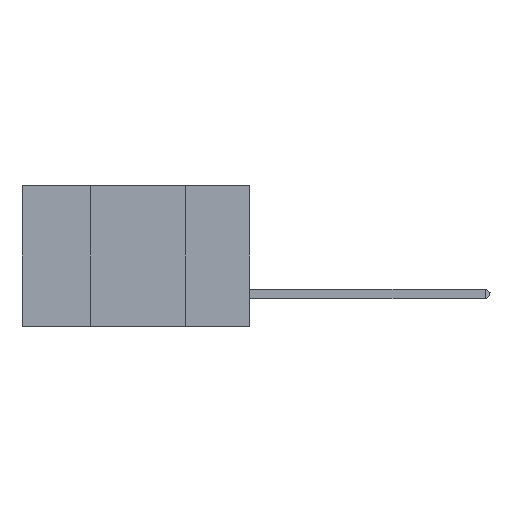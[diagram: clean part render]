
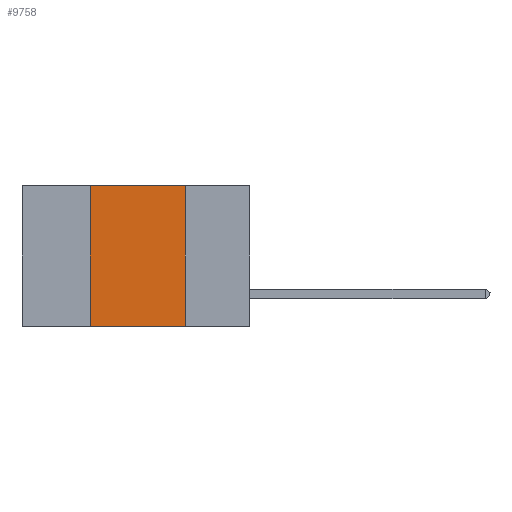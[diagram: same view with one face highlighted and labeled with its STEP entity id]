
A CAD part, left-side view. The second image highlights one B-rep face of the part: STEP entity #9758.
In plain terms, the highlighted planar face has unit normal (-1, 0, 0).
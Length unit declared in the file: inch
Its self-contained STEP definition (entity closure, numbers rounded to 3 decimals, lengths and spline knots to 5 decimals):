
#1117 = DIRECTION ( 'NONE',  ( 0., -1., 0. ) ) ;
#2563 = DIRECTION ( 'NONE',  ( 1., 0., 0. ) ) ;
#5651 = EDGE_CURVE ( 'NONE', #31371, #19098, #8534, .T. ) ;
#6419 = ORIENTED_EDGE ( 'NONE', *, *, #32603, .F. ) ;
#7339 = EDGE_CURVE ( 'NONE', #34856, #31371, #29170, .T. ) ;
#8534 = LINE ( 'NONE', #19761, #28905 ) ;
#9626 = FACE_OUTER_BOUND ( 'NONE', #15199, .T. ) ;
#9758 = ADVANCED_FACE ( 'NONE', ( #9626 ), #15327, .F. ) ;
#10983 = CARTESIAN_POINT ( 'NONE',  ( 0., 0.17, -0.37 ) ) ;
#11455 = CARTESIAN_POINT ( 'NONE',  ( 0., 0.42, 0. ) ) ;
#12037 = CARTESIAN_POINT ( 'NONE',  ( 0., 0.6, 0. ) ) ;
#12449 = DIRECTION ( 'NONE',  ( 0., 0., -1. ) ) ;
#13254 = LINE ( 'NONE', #16245, #29549 ) ;
#15199 = EDGE_LOOP ( 'NONE', ( #35766, #40842, #6419, #17055 ) ) ;
#15327 = PLANE ( 'NONE',  #24045 ) ;
#15795 = VERTEX_POINT ( 'NONE', #33025 ) ;
#16245 = CARTESIAN_POINT ( 'NONE',  ( 0., 0.42, 0. ) ) ;
#17055 = ORIENTED_EDGE ( 'NONE', *, *, #34862, .T. ) ;
#17688 = CARTESIAN_POINT ( 'NONE',  ( 0., 0.6, 0. ) ) ;
#19098 = VERTEX_POINT ( 'NONE', #10983 ) ;
#19761 = CARTESIAN_POINT ( 'NONE',  ( 0., 0.17, 0. ) ) ;
#20621 = DIRECTION ( 'NONE',  ( 0., 0., -1. ) ) ;
#24045 = AXIS2_PLACEMENT_3D ( 'NONE', #12037, #2563, #12449 ) ;
#24137 = DIRECTION ( 'NONE',  ( 0., -1., 0. ) ) ;
#28905 = VECTOR ( 'NONE', #20621, 39.37008 ) ;
#29170 = LINE ( 'NONE', #17688, #41413 ) ;
#29549 = VECTOR ( 'NONE', #42284, 39.37008 ) ;
#30669 = CARTESIAN_POINT ( 'NONE',  ( 0., 0.6, -0.37 ) ) ;
#31371 = VERTEX_POINT ( 'NONE', #32953 ) ;
#32603 = EDGE_CURVE ( 'NONE', #15795, #34856, #13254, .T. ) ;
#32953 = CARTESIAN_POINT ( 'NONE',  ( 0., 0.17, 0. ) ) ;
#33025 = CARTESIAN_POINT ( 'NONE',  ( 0., 0.42, -0.37 ) ) ;
#34856 = VERTEX_POINT ( 'NONE', #11455 ) ;
#34862 = EDGE_CURVE ( 'NONE', #15795, #19098, #37520, .T. ) ;
#35766 = ORIENTED_EDGE ( 'NONE', *, *, #5651, .F. ) ;
#37520 = LINE ( 'NONE', #30669, #39535 ) ;
#39535 = VECTOR ( 'NONE', #24137, 39.37008 ) ;
#40842 = ORIENTED_EDGE ( 'NONE', *, *, #7339, .F. ) ;
#41413 = VECTOR ( 'NONE', #1117, 39.37008 ) ;
#42284 = DIRECTION ( 'NONE',  ( 0., 0., 1. ) ) ;
